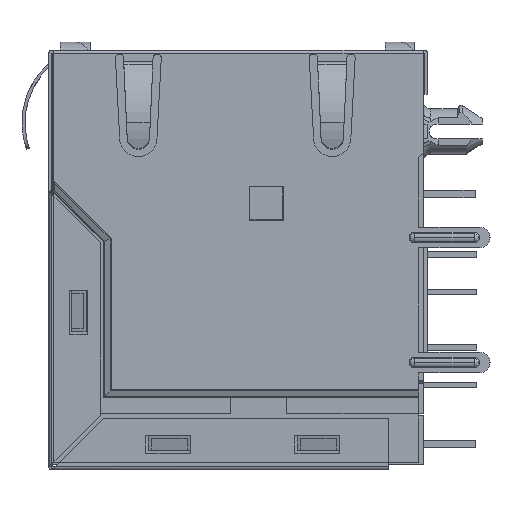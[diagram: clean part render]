
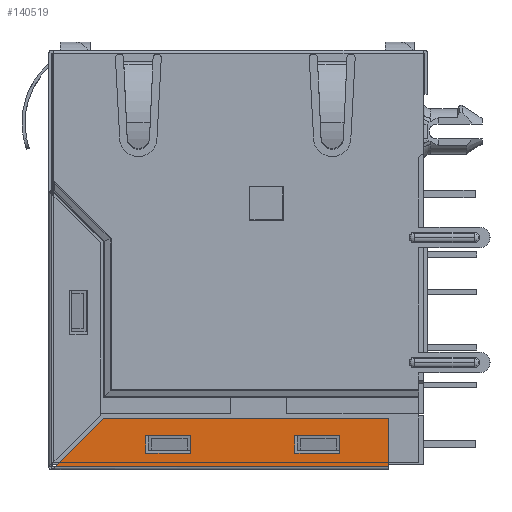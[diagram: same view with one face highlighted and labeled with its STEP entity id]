
A CAD part, left-side view. The second image highlights one B-rep face of the part: STEP entity #140519.
In plain terms, the highlighted planar face has unit normal (-1, 0, 0).
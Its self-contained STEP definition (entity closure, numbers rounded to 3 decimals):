
#1361 = CARTESIAN_POINT ( 'NONE',  ( -31.875, -3.835, -26.78 ) ) ;
#3467 = ORIENTED_EDGE ( 'NONE', *, *, #59342, .T. ) ;
#6857 = EDGE_CURVE ( 'NONE', #81083, #136653, #39101, .T. ) ;
#9596 = VERTEX_POINT ( 'NONE', #144224 ) ;
#11502 = EDGE_CURVE ( 'NONE', #87896, #29399, #79052, .T. ) ;
#13771 = CARTESIAN_POINT ( 'NONE',  ( -31.875, -10.135, -27.67 ) ) ;
#17262 = B_SPLINE_CURVE_WITH_KNOTS ( 'NONE', 1,
 ( #128823, #105515 ),
 .UNSPECIFIED., .F., .F.,
 ( 2, 2 ),
 ( 0., 1. ),
 .UNSPECIFIED. ) ;
#18331 = CARTESIAN_POINT ( 'NONE',  ( -31.875, -10.135, -27.67 ) ) ;
#18772 = CARTESIAN_POINT ( 'NONE',  ( -31.875, 6.165, -26.78 ) ) ;
#24292 = CARTESIAN_POINT ( 'NONE',  ( -31.875, 6.165, -25.58 ) ) ;
#24856 = B_SPLINE_CURVE_WITH_KNOTS ( 'NONE', 1,
 ( #64684, #145515 ),
 .UNSPECIFIED., .F., .F.,
 ( 2, 2 ),
 ( 0., 1. ),
 .UNSPECIFIED. ) ;
#25483 = ORIENTED_EDGE ( 'NONE', *, *, #101811, .T. ) ;
#27937 = EDGE_CURVE ( 'NONE', #74526, #57492, #110360, .T. ) ;
#28204 = EDGE_CURVE ( 'NONE', #9596, #35004, #76171, .T. ) ;
#29040 = EDGE_CURVE ( 'NONE', #57492, #37061, #130777, .T. ) ;
#29399 = VERTEX_POINT ( 'NONE', #79495 ) ;
#31262 = CARTESIAN_POINT ( 'NONE',  ( -31.875, -6.835, -26.78 ) ) ;
#33151 = AXIS2_PLACEMENT_3D ( 'NONE', #40900, #76366, #122367 ) ;
#35004 = VERTEX_POINT ( 'NONE', #58720 ) ;
#35436 = CARTESIAN_POINT ( 'NONE',  ( -31.875, -10.135, -24.43 ) ) ;
#37061 = VERTEX_POINT ( 'NONE', #56053 ) ;
#38894 = CARTESIAN_POINT ( 'NONE',  ( -31.875, 6.165, -26.78 ) ) ;
#39101 = B_SPLINE_CURVE_WITH_KNOTS ( 'NONE', 1,
 ( #91366, #67150 ),
 .UNSPECIFIED., .F., .F.,
 ( 2, 2 ),
 ( 0., 1. ),
 .UNSPECIFIED. ) ;
#40659 = ORIENTED_EDGE ( 'NONE', *, *, #11502, .F. ) ;
#40729 = ORIENTED_EDGE ( 'NONE', *, *, #92142, .F. ) ;
#40900 = CARTESIAN_POINT ( 'NONE',  ( -31.875, 12.693, -27.766 ) ) ;
#45522 = EDGE_LOOP ( 'NONE', ( #40729, #85582, #148998, #40659 ) ) ;
#56032 = EDGE_LOOP ( 'NONE', ( #85590, #3467, #107505, #77561 ) ) ;
#56053 = CARTESIAN_POINT ( 'NONE',  ( -31.875, 6.165, -25.58 ) ) ;
#57323 = B_SPLINE_CURVE_WITH_KNOTS ( 'NONE', 1,
 ( #111945, #18331 ),
 .UNSPECIFIED., .F., .F.,
 ( 2, 2 ),
 ( 0., 1. ),
 .UNSPECIFIED. ) ;
#57492 = VERTEX_POINT ( 'NONE', #128138 ) ;
#58720 = CARTESIAN_POINT ( 'NONE',  ( -31.875, -6.835, -26.78 ) ) ;
#58846 = ORIENTED_EDGE ( 'NONE', *, *, #27937, .T. ) ;
#59342 = EDGE_CURVE ( 'NONE', #126770, #9596, #17262, .T. ) ;
#64246 = PLANE ( 'NONE',  #33151 ) ;
#64684 = CARTESIAN_POINT ( 'NONE',  ( -31.875, 3.165, -25.58 ) ) ;
#66315 = EDGE_LOOP ( 'NONE', ( #90590, #25483, #91865, #58846 ) ) ;
#67150 = CARTESIAN_POINT ( 'NONE',  ( -31.875, -10.135, -27.67 ) ) ;
#68416 = CARTESIAN_POINT ( 'NONE',  ( -31.875, 12.245, -27.67 ) ) ;
#68707 = CARTESIAN_POINT ( 'NONE',  ( -31.875, -6.835, -26.78 ) ) ;
#70938 = CARTESIAN_POINT ( 'NONE',  ( -31.875, 3.165, -25.58 ) ) ;
#71806 = CARTESIAN_POINT ( 'NONE',  ( -31.875, -3.835, -25.58 ) ) ;
#74526 = VERTEX_POINT ( 'NONE', #131664 ) ;
#75288 = EDGE_CURVE ( 'NONE', #35004, #125189, #96965, .T. ) ;
#76171 = B_SPLINE_CURVE_WITH_KNOTS ( 'NONE', 1,
 ( #79795, #68707 ),
 .UNSPECIFIED., .F., .F.,
 ( 2, 2 ),
 ( 0., 1. ),
 .UNSPECIFIED. ) ;
#76366 = DIRECTION ( 'NONE',  ( -1., 0., 0. ) ) ;
#77561 = ORIENTED_EDGE ( 'NONE', *, *, #75288, .T. ) ;
#79052 = B_SPLINE_CURVE_WITH_KNOTS ( 'NONE', 1,
 ( #94126, #35436 ),
 .UNSPECIFIED., .F., .F.,
 ( 2, 2 ),
 ( 0., 1. ),
 .UNSPECIFIED. ) ;
#79495 = CARTESIAN_POINT ( 'NONE',  ( -31.875, -10.135, -24.43 ) ) ;
#79795 = CARTESIAN_POINT ( 'NONE',  ( -31.875, -6.835, -25.58 ) ) ;
#81083 = VERTEX_POINT ( 'NONE', #68416 ) ;
#85582 = ORIENTED_EDGE ( 'NONE', *, *, #6857, .T. ) ;
#85590 = ORIENTED_EDGE ( 'NONE', *, *, #115973, .T. ) ;
#86016 = CARTESIAN_POINT ( 'NONE',  ( -31.875, 3.165, -26.78 ) ) ;
#87896 = VERTEX_POINT ( 'NONE', #139830 ) ;
#88038 = B_SPLINE_CURVE_WITH_KNOTS ( 'NONE', 1,
 ( #24292, #70938 ),
 .UNSPECIFIED., .F., .F.,
 ( 2, 2 ),
 ( 0., 1. ),
 .UNSPECIFIED. ) ;
#90590 = ORIENTED_EDGE ( 'NONE', *, *, #29040, .T. ) ;
#91366 = CARTESIAN_POINT ( 'NONE',  ( -31.875, 12.245, -27.67 ) ) ;
#91865 = ORIENTED_EDGE ( 'NONE', *, *, #104863, .T. ) ;
#92142 = EDGE_CURVE ( 'NONE', #81083, #87896, #100610, .T. ) ;
#92841 = CARTESIAN_POINT ( 'NONE',  ( -31.875, -3.835, -25.58 ) ) ;
#94126 = CARTESIAN_POINT ( 'NONE',  ( -31.875, 9.005, -24.43 ) ) ;
#96965 = B_SPLINE_CURVE_WITH_KNOTS ( 'NONE', 1,
 ( #31262, #112211 ),
 .UNSPECIFIED., .F., .F.,
 ( 2, 2 ),
 ( 0., 1. ),
 .UNSPECIFIED. ) ;
#100610 = B_SPLINE_CURVE_WITH_KNOTS ( 'NONE', 1,
 ( #102778, #137716 ),
 .UNSPECIFIED., .F., .F.,
 ( 2, 2 ),
 ( 0., 1. ),
 .UNSPECIFIED. ) ;
#101811 = EDGE_CURVE ( 'NONE', #37061, #108646, #88038, .T. ) ;
#102732 = FACE_OUTER_BOUND ( 'NONE', #45522, .T. ) ;
#102778 = CARTESIAN_POINT ( 'NONE',  ( -31.875, 12.245, -27.67 ) ) ;
#104863 = EDGE_CURVE ( 'NONE', #108646, #74526, #24856, .T. ) ;
#105515 = CARTESIAN_POINT ( 'NONE',  ( -31.875, -6.835, -25.58 ) ) ;
#105639 = CARTESIAN_POINT ( 'NONE',  ( -31.875, -3.835, -26.78 ) ) ;
#107505 = ORIENTED_EDGE ( 'NONE', *, *, #28204, .T. ) ;
#108436 = EDGE_CURVE ( 'NONE', #29399, #136653, #57323, .T. ) ;
#108646 = VERTEX_POINT ( 'NONE', #127599 ) ;
#110360 = B_SPLINE_CURVE_WITH_KNOTS ( 'NONE', 1,
 ( #86016, #38894 ),
 .UNSPECIFIED., .F., .F.,
 ( 2, 2 ),
 ( 0., 1. ),
 .UNSPECIFIED. ) ;
#111945 = CARTESIAN_POINT ( 'NONE',  ( -31.875, -10.135, -24.43 ) ) ;
#112211 = CARTESIAN_POINT ( 'NONE',  ( -31.875, -3.835, -26.78 ) ) ;
#115973 = EDGE_CURVE ( 'NONE', #125189, #126770, #129602, .T. ) ;
#122367 = DIRECTION ( 'NONE',  ( 0., -1., 0. ) ) ;
#125189 = VERTEX_POINT ( 'NONE', #105639 ) ;
#126770 = VERTEX_POINT ( 'NONE', #92841 ) ;
#127599 = CARTESIAN_POINT ( 'NONE',  ( -31.875, 3.165, -25.58 ) ) ;
#128015 = FACE_BOUND ( 'NONE', #66315, .T. ) ;
#128138 = CARTESIAN_POINT ( 'NONE',  ( -31.875, 6.165, -26.78 ) ) ;
#128823 = CARTESIAN_POINT ( 'NONE',  ( -31.875, -3.835, -25.58 ) ) ;
#129602 = B_SPLINE_CURVE_WITH_KNOTS ( 'NONE', 1,
 ( #1361, #71806 ),
 .UNSPECIFIED., .F., .F.,
 ( 2, 2 ),
 ( 0., 1. ),
 .UNSPECIFIED. ) ;
#130777 = B_SPLINE_CURVE_WITH_KNOTS ( 'NONE', 1,
 ( #18772, #134704 ),
 .UNSPECIFIED., .F., .F.,
 ( 2, 2 ),
 ( 0., 1. ),
 .UNSPECIFIED. ) ;
#131664 = CARTESIAN_POINT ( 'NONE',  ( -31.875, 3.165, -26.78 ) ) ;
#134704 = CARTESIAN_POINT ( 'NONE',  ( -31.875, 6.165, -25.58 ) ) ;
#135291 = FACE_BOUND ( 'NONE', #56032, .T. ) ;
#136653 = VERTEX_POINT ( 'NONE', #13771 ) ;
#137716 = CARTESIAN_POINT ( 'NONE',  ( -31.875, 9.005, -24.43 ) ) ;
#139830 = CARTESIAN_POINT ( 'NONE',  ( -31.875, 9.005, -24.43 ) ) ;
#140519 = ADVANCED_FACE ( 'NONE', ( #102732, #128015, #135291 ), #64246, .T. ) ;
#144224 = CARTESIAN_POINT ( 'NONE',  ( -31.875, -6.835, -25.58 ) ) ;
#145515 = CARTESIAN_POINT ( 'NONE',  ( -31.875, 3.165, -26.78 ) ) ;
#148998 = ORIENTED_EDGE ( 'NONE', *, *, #108436, .F. ) ;
